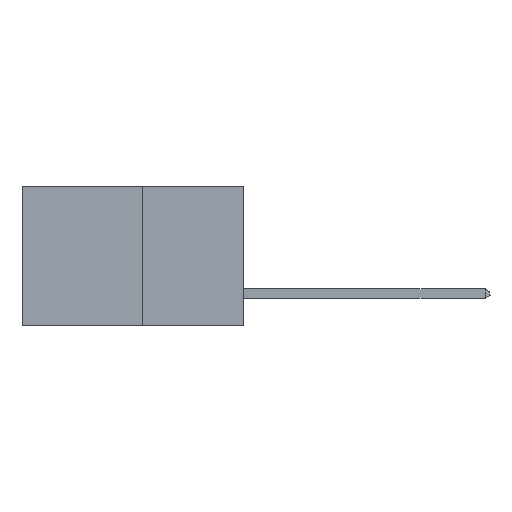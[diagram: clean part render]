
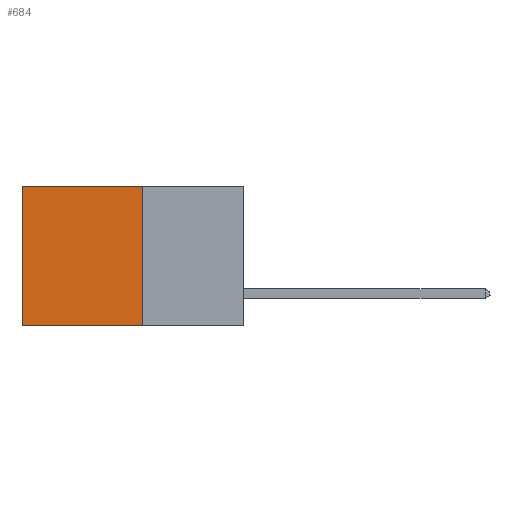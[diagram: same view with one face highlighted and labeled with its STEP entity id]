
A CAD part, left-side view. The second image highlights one B-rep face of the part: STEP entity #684.
In plain terms, the highlighted planar face has unit normal (-1, 0, 0).
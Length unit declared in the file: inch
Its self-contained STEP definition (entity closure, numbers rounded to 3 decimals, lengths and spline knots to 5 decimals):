
#563 = AXIS2_PLACEMENT_3D ( 'NONE', #4286, #2273, #2264 ) ;
#579 = LINE ( 'NONE', #8370, #6168 ) ;
#684 = ADVANCED_FACE ( 'NONE', ( #2749 ), #4262, .F. ) ;
#736 = CARTESIAN_POINT ( 'NONE',  ( 0.277, 0.27, -0.37 ) ) ;
#931 = CARTESIAN_POINT ( 'NONE',  ( 0.277, 0.27, 0. ) ) ;
#1791 = ORIENTED_EDGE ( 'NONE', *, *, #3889, .T. ) ;
#2264 = DIRECTION ( 'NONE',  ( 0., 0., -1. ) ) ;
#2273 = DIRECTION ( 'NONE',  ( 1., 0., 0. ) ) ;
#2555 = EDGE_CURVE ( 'NONE', #4919, #4759, #579, .T. ) ;
#2558 = VECTOR ( 'NONE', #5821, 39.37008 ) ;
#2749 = FACE_OUTER_BOUND ( 'NONE', #6048, .T. ) ;
#2909 = CARTESIAN_POINT ( 'NONE',  ( 0.277, 0.59, 0. ) ) ;
#3039 = EDGE_CURVE ( 'NONE', #5101, #6156, #4624, .T. ) ;
#3572 = ORIENTED_EDGE ( 'NONE', *, *, #2555, .T. ) ;
#3687 = CARTESIAN_POINT ( 'NONE',  ( 0.277, 0.59, -0.37 ) ) ;
#3889 = EDGE_CURVE ( 'NONE', #5101, #4919, #5105, .T. ) ;
#3917 = EDGE_CURVE ( 'NONE', #6156, #4759, #8019, .T. ) ;
#4262 = PLANE ( 'NONE',  #563 ) ;
#4286 = CARTESIAN_POINT ( 'NONE',  ( 0.277, 0.27, -0.37 ) ) ;
#4624 = LINE ( 'NONE', #5915, #2558 ) ;
#4759 = VERTEX_POINT ( 'NONE', #3687 ) ;
#4899 = VECTOR ( 'NONE', #8448, 39.37008 ) ;
#4919 = VERTEX_POINT ( 'NONE', #2909 ) ;
#5101 = VERTEX_POINT ( 'NONE', #931 ) ;
#5105 = LINE ( 'NONE', #8555, #6616 ) ;
#5331 = ORIENTED_EDGE ( 'NONE', *, *, #3917, .F. ) ;
#5821 = DIRECTION ( 'NONE',  ( 0., 0., -1. ) ) ;
#5915 = CARTESIAN_POINT ( 'NONE',  ( 0.277, 0.27, -0.37 ) ) ;
#6048 = EDGE_LOOP ( 'NONE', ( #3572, #5331, #8549, #1791 ) ) ;
#6156 = VERTEX_POINT ( 'NONE', #736 ) ;
#6168 = VECTOR ( 'NONE', #8728, 39.37008 ) ;
#6616 = VECTOR ( 'NONE', #8554, 39.37008 ) ;
#8019 = LINE ( 'NONE', #8525, #4899 ) ;
#8370 = CARTESIAN_POINT ( 'NONE',  ( 0.277, 0.59, -0.37 ) ) ;
#8448 = DIRECTION ( 'NONE',  ( 0., 1., 0. ) ) ;
#8525 = CARTESIAN_POINT ( 'NONE',  ( 0.277, 0.27, -0.37 ) ) ;
#8549 = ORIENTED_EDGE ( 'NONE', *, *, #3039, .F. ) ;
#8554 = DIRECTION ( 'NONE',  ( 0., 1., 0. ) ) ;
#8555 = CARTESIAN_POINT ( 'NONE',  ( 0.277, 0.27, 0. ) ) ;
#8728 = DIRECTION ( 'NONE',  ( 0., 0., -1. ) ) ;
